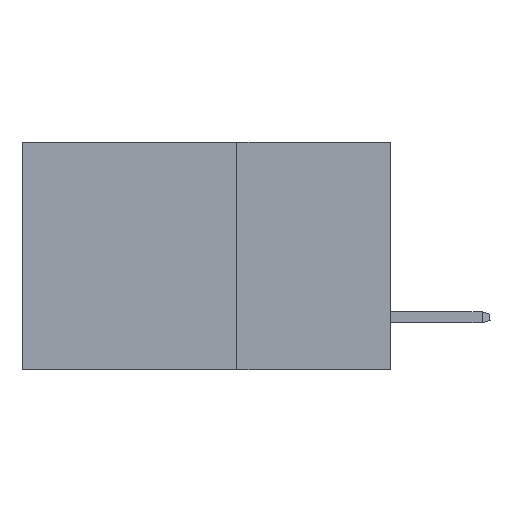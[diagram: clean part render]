
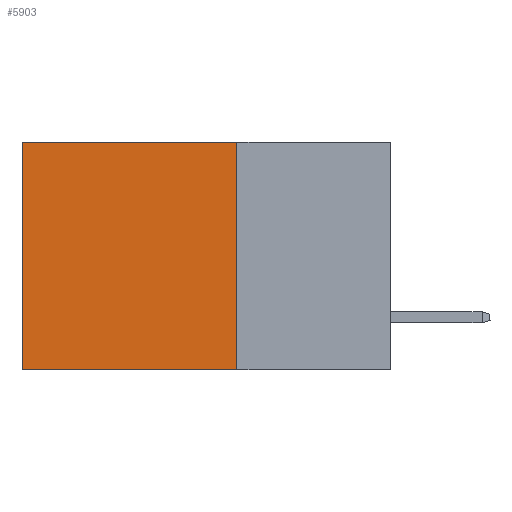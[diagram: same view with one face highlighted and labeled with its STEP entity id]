
A CAD part, left-side view. The second image highlights one B-rep face of the part: STEP entity #5903.
In plain terms, the highlighted planar face has unit normal (-1, 0, 0).
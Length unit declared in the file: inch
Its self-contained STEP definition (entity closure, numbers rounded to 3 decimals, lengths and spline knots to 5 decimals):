
#544 = AXIS2_PLACEMENT_3D ( 'NONE', #7258, #16197, #8593 ) ;
#2015 = EDGE_CURVE ( 'NONE', #13843, #9138, #13734, .T. ) ;
#2709 = DIRECTION ( 'NONE',  ( 0., 1., 0. ) ) ;
#2784 = DIRECTION ( 'NONE',  ( 0., 0., -1. ) ) ;
#2815 = VECTOR ( 'NONE', #14783, 39.37008 ) ;
#3265 = VECTOR ( 'NONE', #13822, 39.37008 ) ;
#4160 = ORIENTED_EDGE ( 'NONE', *, *, #5767, .F. ) ;
#4193 = ORIENTED_EDGE ( 'NONE', *, *, #2015, .F. ) ;
#4374 = CARTESIAN_POINT ( 'NONE',  ( 0.2875, 0.25, 0. ) ) ;
#5063 = LINE ( 'NONE', #9304, #8599 ) ;
#5221 = CARTESIAN_POINT ( 'NONE',  ( 0.2875, 0.25, -0.37 ) ) ;
#5767 = EDGE_CURVE ( 'NONE', #14217, #13843, #6332, .T. ) ;
#5903 = ADVANCED_FACE ( 'NONE', ( #14261 ), #11138, .F. ) ;
#6038 = ORIENTED_EDGE ( 'NONE', *, *, #11084, .T. ) ;
#6297 = EDGE_CURVE ( 'NONE', #14217, #15530, #5063, .T. ) ;
#6332 = LINE ( 'NONE', #4374, #2815 ) ;
#7258 = CARTESIAN_POINT ( 'NONE',  ( 0.2875, 0.25, 0. ) ) ;
#7483 = VECTOR ( 'NONE', #2784, 39.37008 ) ;
#7770 = ORIENTED_EDGE ( 'NONE', *, *, #6297, .T. ) ;
#8593 = DIRECTION ( 'NONE',  ( 0., 0., -1. ) ) ;
#8599 = VECTOR ( 'NONE', #2709, 39.37008 ) ;
#9138 = VERTEX_POINT ( 'NONE', #12216 ) ;
#9304 = CARTESIAN_POINT ( 'NONE',  ( 0.2875, 0.25, 0. ) ) ;
#11084 = EDGE_CURVE ( 'NONE', #15530, #9138, #11358, .T. ) ;
#11138 = PLANE ( 'NONE',  #544 ) ;
#11358 = LINE ( 'NONE', #15710, #7483 ) ;
#11459 = CARTESIAN_POINT ( 'NONE',  ( 0.2875, 0.25, -0.37 ) ) ;
#12216 = CARTESIAN_POINT ( 'NONE',  ( 0.2875, 0.6, -0.37 ) ) ;
#13734 = LINE ( 'NONE', #11459, #3265 ) ;
#13822 = DIRECTION ( 'NONE',  ( 0., 1., 0. ) ) ;
#13843 = VERTEX_POINT ( 'NONE', #5221 ) ;
#14082 = CARTESIAN_POINT ( 'NONE',  ( 0.2875, 0.25, 0. ) ) ;
#14217 = VERTEX_POINT ( 'NONE', #14082 ) ;
#14261 = FACE_OUTER_BOUND ( 'NONE', #15644, .T. ) ;
#14783 = DIRECTION ( 'NONE',  ( 0., 0., -1. ) ) ;
#15530 = VERTEX_POINT ( 'NONE', #16093 ) ;
#15644 = EDGE_LOOP ( 'NONE', ( #6038, #4193, #4160, #7770 ) ) ;
#15710 = CARTESIAN_POINT ( 'NONE',  ( 0.2875, 0.6, 0. ) ) ;
#16093 = CARTESIAN_POINT ( 'NONE',  ( 0.2875, 0.6, 0. ) ) ;
#16197 = DIRECTION ( 'NONE',  ( 1., 0., 0. ) ) ;
